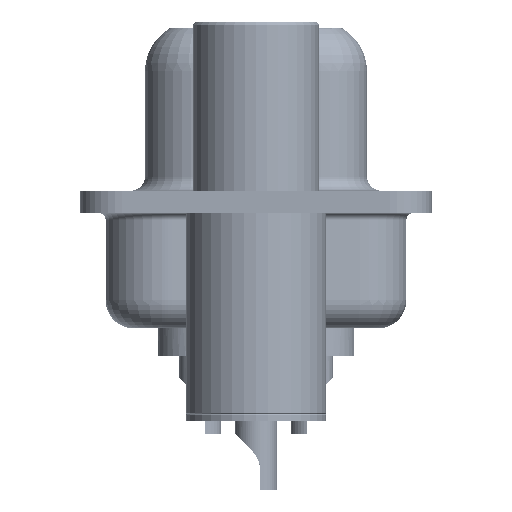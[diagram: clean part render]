
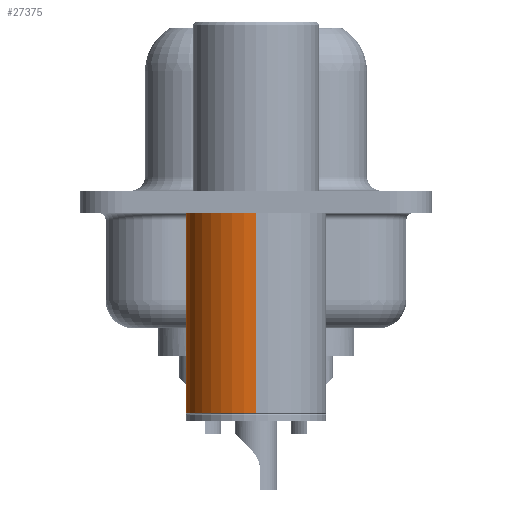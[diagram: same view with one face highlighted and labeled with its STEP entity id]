
A CAD part, left-side view. The second image highlights one B-rep face of the part: STEP entity #27375.
In plain terms, the highlighted cylindrical face has radius 2.5 mm (diameter 5 mm), a partial arc.
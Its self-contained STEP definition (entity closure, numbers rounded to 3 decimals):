
#3921 = ORIENTED_EDGE ( 'NONE', *, *, #7160, .F. ) ;
#4565 = EDGE_LOOP ( 'NONE', ( #33196, #8296, #34698, #3921 ) ) ;
#4762 = AXIS2_PLACEMENT_3D ( 'NONE', #13517, #16544, #19949 ) ;
#5459 = CARTESIAN_POINT ( 'NONE',  ( 0., 0., -7.525 ) ) ;
#6799 = DIRECTION ( 'NONE',  ( 0., 0., 1. ) ) ;
#7160 = EDGE_CURVE ( 'NONE', #26501, #8970, #22705, .T. ) ;
#7733 = CARTESIAN_POINT ( 'NONE',  ( 2.5, 0., -0.4 ) ) ;
#7997 = DIRECTION ( 'NONE',  ( 0., 0., 1. ) ) ;
#8296 = ORIENTED_EDGE ( 'NONE', *, *, #34291, .T. ) ;
#8353 = DIRECTION ( 'NONE',  ( 1., 0., 0. ) ) ;
#8970 = VERTEX_POINT ( 'NONE', #7733 ) ;
#10684 = FACE_OUTER_BOUND ( 'NONE', #4565, .T. ) ;
#11575 = CARTESIAN_POINT ( 'NONE',  ( 0., 0., -0.4 ) ) ;
#13517 = CARTESIAN_POINT ( 'NONE',  ( 0., 0., 0.581 ) ) ;
#15354 = VECTOR ( 'NONE', #6799, 1000. ) ;
#15848 = EDGE_CURVE ( 'NONE', #26501, #38480, #21464, .T. ) ;
#16474 = LINE ( 'NONE', #34847, #15354 ) ;
#16544 = DIRECTION ( 'NONE',  ( 0., 0., 1. ) ) ;
#17030 = CARTESIAN_POINT ( 'NONE',  ( 2.5, 0., -7.525 ) ) ;
#17969 = DIRECTION ( 'NONE',  ( 0., 0., 1. ) ) ;
#19949 = DIRECTION ( 'NONE',  ( 1., 0., 0. ) ) ;
#21464 = CIRCLE ( 'NONE', #23413, 2.5 ) ;
#21774 = CARTESIAN_POINT ( 'NONE',  ( -2.5, 0., -7.525 ) ) ;
#22705 = LINE ( 'NONE', #23517, #25577 ) ;
#23413 = AXIS2_PLACEMENT_3D ( 'NONE', #5459, #17969, #27247 ) ;
#23517 = CARTESIAN_POINT ( 'NONE',  ( 2.5, 0., 0.581 ) ) ;
#25100 = VERTEX_POINT ( 'NONE', #35800 ) ;
#25577 = VECTOR ( 'NONE', #7997, 1000. ) ;
#26501 = VERTEX_POINT ( 'NONE', #17030 ) ;
#27247 = DIRECTION ( 'NONE',  ( 1., 0., 0. ) ) ;
#27375 = ADVANCED_FACE ( 'NONE', ( #10684 ), #29252, .T. ) ;
#27413 = CIRCLE ( 'NONE', #39668, 2.5 ) ;
#29252 = CYLINDRICAL_SURFACE ( 'NONE', #4762, 2.5 ) ;
#30369 = EDGE_CURVE ( 'NONE', #8970, #25100, #27413, .T. ) ;
#33175 = DIRECTION ( 'NONE',  ( 0., 0., 1. ) ) ;
#33196 = ORIENTED_EDGE ( 'NONE', *, *, #15848, .T. ) ;
#34291 = EDGE_CURVE ( 'NONE', #38480, #25100, #16474, .T. ) ;
#34698 = ORIENTED_EDGE ( 'NONE', *, *, #30369, .F. ) ;
#34847 = CARTESIAN_POINT ( 'NONE',  ( -2.5, 0., 0.581 ) ) ;
#35800 = CARTESIAN_POINT ( 'NONE',  ( -2.5, 0., -0.4 ) ) ;
#38480 = VERTEX_POINT ( 'NONE', #21774 ) ;
#39668 = AXIS2_PLACEMENT_3D ( 'NONE', #11575, #33175, #8353 ) ;
